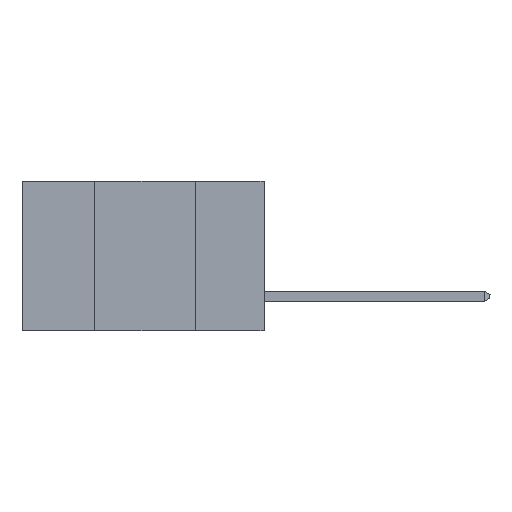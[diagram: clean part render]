
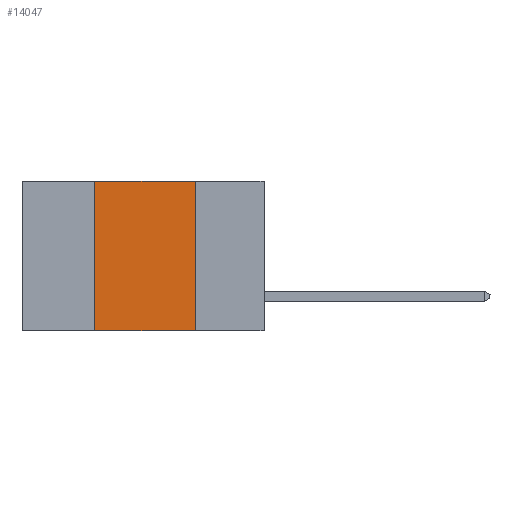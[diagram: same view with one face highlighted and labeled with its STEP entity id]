
A CAD part, left-side view. The second image highlights one B-rep face of the part: STEP entity #14047.
In plain terms, the highlighted planar face has unit normal (-1, 0, 0).
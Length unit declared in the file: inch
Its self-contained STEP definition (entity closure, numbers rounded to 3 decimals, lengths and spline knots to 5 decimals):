
#965 = DIRECTION ( 'NONE',  ( 0., -1., 0. ) ) ;
#2251 = DIRECTION ( 'NONE',  ( 0., 0., -1. ) ) ;
#2255 = ORIENTED_EDGE ( 'NONE', *, *, #18002, .F. ) ;
#2571 = CARTESIAN_POINT ( 'NONE',  ( 0., 0.6, -0.37 ) ) ;
#2834 = DIRECTION ( 'NONE',  ( 0., -1., 0. ) ) ;
#3136 = VERTEX_POINT ( 'NONE', #15628 ) ;
#4922 = VECTOR ( 'NONE', #2834, 39.37008 ) ;
#5738 = ORIENTED_EDGE ( 'NONE', *, *, #9365, .T. ) ;
#5864 = ORIENTED_EDGE ( 'NONE', *, *, #18268, .F. ) ;
#5945 = LINE ( 'NONE', #17808, #4922 ) ;
#6012 = VECTOR ( 'NONE', #965, 39.37008 ) ;
#7190 = CARTESIAN_POINT ( 'NONE',  ( 0., 0.6, 0. ) ) ;
#8245 = LINE ( 'NONE', #20094, #12111 ) ;
#8312 = VERTEX_POINT ( 'NONE', #18459 ) ;
#9365 = EDGE_CURVE ( 'NONE', #3136, #15111, #10411, .T. ) ;
#10411 = LINE ( 'NONE', #2571, #6012 ) ;
#11853 = VECTOR ( 'NONE', #16223, 39.37008 ) ;
#12111 = VECTOR ( 'NONE', #16668, 39.37008 ) ;
#12772 = EDGE_LOOP ( 'NONE', ( #5864, #19267, #2255, #5738 ) ) ;
#12792 = AXIS2_PLACEMENT_3D ( 'NONE', #7190, #15530, #2251 ) ;
#13023 = CARTESIAN_POINT ( 'NONE',  ( 0., 0.17, 0. ) ) ;
#13489 = VERTEX_POINT ( 'NONE', #13023 ) ;
#14047 = ADVANCED_FACE ( 'NONE', ( #14182 ), #17076, .F. ) ;
#14182 = FACE_OUTER_BOUND ( 'NONE', #12772, .T. ) ;
#15111 = VERTEX_POINT ( 'NONE', #16852 ) ;
#15530 = DIRECTION ( 'NONE',  ( 1., 0., 0. ) ) ;
#15628 = CARTESIAN_POINT ( 'NONE',  ( 0., 0.42, -0.37 ) ) ;
#16223 = DIRECTION ( 'NONE',  ( 0., 0., 1. ) ) ;
#16668 = DIRECTION ( 'NONE',  ( 0., 0., -1. ) ) ;
#16852 = CARTESIAN_POINT ( 'NONE',  ( 0., 0.17, -0.37 ) ) ;
#17076 = PLANE ( 'NONE',  #12792 ) ;
#17319 = EDGE_CURVE ( 'NONE', #8312, #13489, #5945, .T. ) ;
#17808 = CARTESIAN_POINT ( 'NONE',  ( 0., 0.6, 0. ) ) ;
#17909 = CARTESIAN_POINT ( 'NONE',  ( 0., 0.42, 0. ) ) ;
#18002 = EDGE_CURVE ( 'NONE', #3136, #8312, #20711, .T. ) ;
#18268 = EDGE_CURVE ( 'NONE', #13489, #15111, #8245, .T. ) ;
#18459 = CARTESIAN_POINT ( 'NONE',  ( 0., 0.42, 0. ) ) ;
#19267 = ORIENTED_EDGE ( 'NONE', *, *, #17319, .F. ) ;
#20094 = CARTESIAN_POINT ( 'NONE',  ( 0., 0.17, 0. ) ) ;
#20711 = LINE ( 'NONE', #17909, #11853 ) ;
